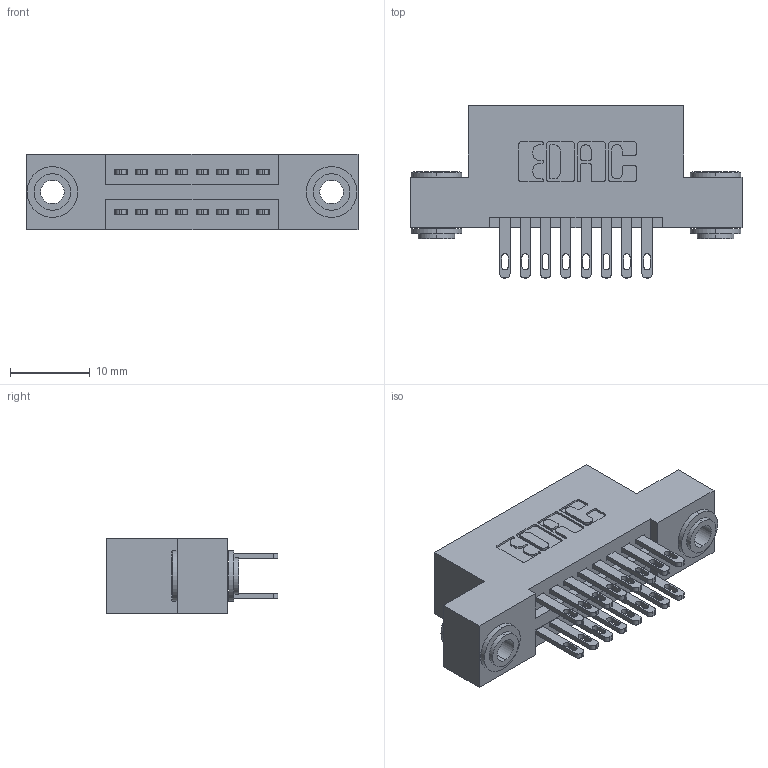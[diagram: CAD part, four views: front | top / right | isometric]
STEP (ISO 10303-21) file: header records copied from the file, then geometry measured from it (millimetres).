
FILE_DESCRIPTION (( 'STEP AP203' ), '1' );
FILE_NAME ('895-016-500-203.STEP', '2020-09-25T04:20:49', ( '' ), ( '' ), 'SwSTEP 2.0', 'SolidWorks 2020', '' );
FILE_SCHEMA (( 'CONFIG_CONTROL_DESIGN' ));
Length unit declared in the file: inch
Products named in the file (4): 345-250-002_345-250-002-102; 845 Part_Flush Mounting Lugs - 0.156 Dia-TH; 895-016-500-203; 345-292-001_345-293-100
Assembly tree (19 placements, depth 2):
  895-016-500-203
    845 Part_Flush Mounting Lugs - 0.156 Dia-TH
    345-292-001_345-293-100  x16
    345-250-002_345-250-002-102  x2
Bounding box: 41.53 x 21.51 x 9.4 mm (x, y, z)
Volume: 3786.9 mm3; surface area: 5307.2 mm2
Topology: 19 solids, 19 shells, 900 faces, 2673 edges, 1778 vertices
Faces by surface type: plane 522, cylinder 370, cone 8
Entity records: 11434 total; most frequent: CARTESIAN_POINT 1923, ORIENTED_EDGE 1850, DIRECTION 1771, EDGE_CURVE 925, VECTOR 733, LINE 733, VERTEX_POINT 614, AXIS2_PLACEMENT_3D 519
